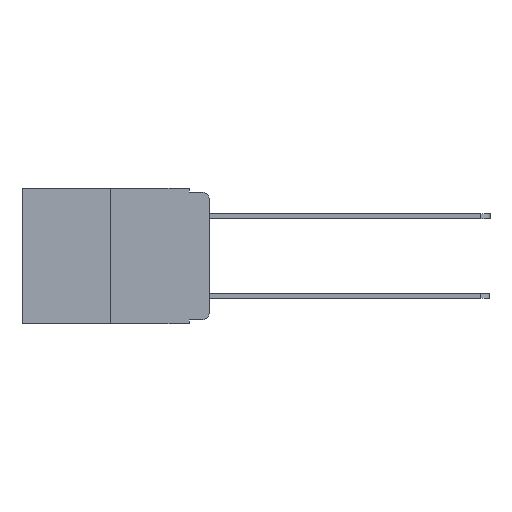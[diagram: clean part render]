
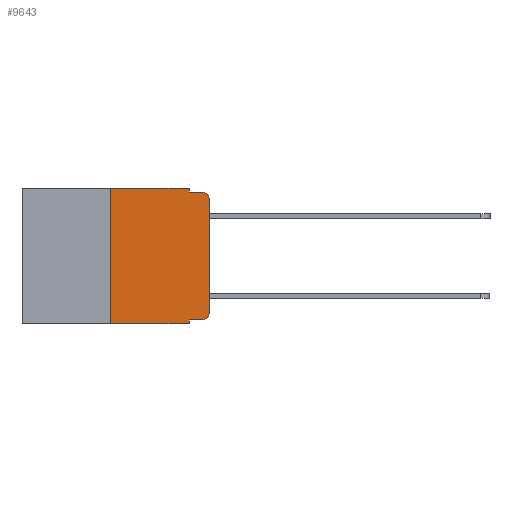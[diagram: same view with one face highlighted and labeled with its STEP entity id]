
A CAD part, left-side view. The second image highlights one B-rep face of the part: STEP entity #9643.
In plain terms, the highlighted planar face has unit normal (-1, 0, 0).
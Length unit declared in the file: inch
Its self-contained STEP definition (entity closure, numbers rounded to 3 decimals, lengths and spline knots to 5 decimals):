
#105 = CARTESIAN_POINT ( 'NONE',  ( 0., 0.051, -0.01 ) ) ;
#121 = CARTESIAN_POINT ( 'NONE',  ( 0., 0., -0.03 ) ) ;
#303 = CARTESIAN_POINT ( 'NONE',  ( 0., 0.02, -0.03 ) ) ;
#440 = CARTESIAN_POINT ( 'NONE',  ( 0., 0., -0.313 ) ) ;
#851 = EDGE_CURVE ( 'NONE', #20736, #8374, #11823, .T. ) ;
#1674 = EDGE_CURVE ( 'NONE', #4114, #20736, #7395, .T. ) ;
#1736 = DIRECTION ( 'NONE',  ( 0., 0., 1. ) ) ;
#1778 = AXIS2_PLACEMENT_3D ( 'NONE', #303, #13627, #2288 ) ;
#2103 = DIRECTION ( 'NONE',  ( 0., -1., 0. ) ) ;
#2275 = CARTESIAN_POINT ( 'NONE',  ( 0., 0.051, -0.01 ) ) ;
#2288 = DIRECTION ( 'NONE',  ( 0., 0., -1. ) ) ;
#2421 = ORIENTED_EDGE ( 'NONE', *, *, #851, .T. ) ;
#2631 = DIRECTION ( 'NONE',  ( 0., 0., -1. ) ) ;
#2921 = EDGE_LOOP ( 'NONE', ( #8877, #15632, #22262, #8631, #10680, #23446, #5410, #3330, #23734, #2421 ) ) ;
#2925 = DIRECTION ( 'NONE',  ( 0., -1., 0. ) ) ;
#3235 = CARTESIAN_POINT ( 'NONE',  ( 0., 0.473, 0. ) ) ;
#3330 = ORIENTED_EDGE ( 'NONE', *, *, #20249, .F. ) ;
#3991 = AXIS2_PLACEMENT_3D ( 'NONE', #8422, #21421, #10295 ) ;
#4114 = VERTEX_POINT ( 'NONE', #14947 ) ;
#4833 = CARTESIAN_POINT ( 'NONE',  ( 0., 0.051, 0. ) ) ;
#5077 = CARTESIAN_POINT ( 'NONE',  ( 0., 0.25, -0.343 ) ) ;
#5410 = ORIENTED_EDGE ( 'NONE', *, *, #15609, .T. ) ;
#5533 = VERTEX_POINT ( 'NONE', #17223 ) ;
#6194 = EDGE_CURVE ( 'NONE', #16056, #20361, #22627, .T. ) ;
#6720 = LINE ( 'NONE', #24196, #20964 ) ;
#7053 = CARTESIAN_POINT ( 'NONE',  ( 0., 0.051, -0.343 ) ) ;
#7395 = LINE ( 'NONE', #8939, #17338 ) ;
#8347 = LINE ( 'NONE', #3235, #18231 ) ;
#8374 = VERTEX_POINT ( 'NONE', #440 ) ;
#8422 = CARTESIAN_POINT ( 'NONE',  ( 0., 0.02, -0.313 ) ) ;
#8479 = CARTESIAN_POINT ( 'NONE',  ( 0., 0.25, 0. ) ) ;
#8631 = ORIENTED_EDGE ( 'NONE', *, *, #10132, .F. ) ;
#8759 = FACE_OUTER_BOUND ( 'NONE', #2921, .T. ) ;
#8877 = ORIENTED_EDGE ( 'NONE', *, *, #9950, .T. ) ;
#8939 = CARTESIAN_POINT ( 'NONE',  ( 0., 0.051, -0.333 ) ) ;
#9478 = EDGE_CURVE ( 'NONE', #22803, #20361, #23287, .T. ) ;
#9643 = ADVANCED_FACE ( 'NONE', ( #8759 ), #10147, .F. ) ;
#9950 = EDGE_CURVE ( 'NONE', #8374, #16056, #6720, .T. ) ;
#10132 = EDGE_CURVE ( 'NONE', #5533, #22803, #17490, .T. ) ;
#10147 = PLANE ( 'NONE',  #22801 ) ;
#10295 = DIRECTION ( 'NONE',  ( 0., 0., -1. ) ) ;
#10396 = CARTESIAN_POINT ( 'NONE',  ( 0., 0.02, -0.333 ) ) ;
#10445 = LINE ( 'NONE', #4833, #11604 ) ;
#10680 = ORIENTED_EDGE ( 'NONE', *, *, #22189, .F. ) ;
#10774 = LINE ( 'NONE', #8479, #20094 ) ;
#10908 = EDGE_CURVE ( 'NONE', #18416, #16336, #10774, .T. ) ;
#11604 = VECTOR ( 'NONE', #17900, 39.37008 ) ;
#11823 = CIRCLE ( 'NONE', #3991, 0.02 ) ;
#12043 = CARTESIAN_POINT ( 'NONE',  ( 0., 0.473, 0. ) ) ;
#13627 = DIRECTION ( 'NONE',  ( -1., 0., 0. ) ) ;
#13941 = DIRECTION ( 'NONE',  ( 1., 0., 0. ) ) ;
#14151 = LINE ( 'NONE', #14222, #23360 ) ;
#14222 = CARTESIAN_POINT ( 'NONE',  ( 0., 0.473, -0.343 ) ) ;
#14449 = VERTEX_POINT ( 'NONE', #7053 ) ;
#14947 = CARTESIAN_POINT ( 'NONE',  ( 0., 0.051, -0.333 ) ) ;
#15609 = EDGE_CURVE ( 'NONE', #18416, #14449, #14151, .T. ) ;
#15632 = ORIENTED_EDGE ( 'NONE', *, *, #6194, .T. ) ;
#16005 = DIRECTION ( 'NONE',  ( 0., 0., 1. ) ) ;
#16056 = VERTEX_POINT ( 'NONE', #121 ) ;
#16336 = VERTEX_POINT ( 'NONE', #19913 ) ;
#16909 = VECTOR ( 'NONE', #19164, 39.37008 ) ;
#17223 = CARTESIAN_POINT ( 'NONE',  ( 0., 0.051, 0. ) ) ;
#17245 = VECTOR ( 'NONE', #2103, 39.37008 ) ;
#17338 = VECTOR ( 'NONE', #21941, 39.37008 ) ;
#17490 = LINE ( 'NONE', #21028, #16909 ) ;
#17900 = DIRECTION ( 'NONE',  ( 0., 0., -1. ) ) ;
#18231 = VECTOR ( 'NONE', #23764, 39.37008 ) ;
#18416 = VERTEX_POINT ( 'NONE', #5077 ) ;
#19164 = DIRECTION ( 'NONE',  ( 0., 0., -1. ) ) ;
#19913 = CARTESIAN_POINT ( 'NONE',  ( 0., 0.25, 0. ) ) ;
#20094 = VECTOR ( 'NONE', #16005, 39.37008 ) ;
#20249 = EDGE_CURVE ( 'NONE', #4114, #14449, #10445, .T. ) ;
#20326 = CARTESIAN_POINT ( 'NONE',  ( 0., 0.02, -0.01 ) ) ;
#20361 = VERTEX_POINT ( 'NONE', #20326 ) ;
#20736 = VERTEX_POINT ( 'NONE', #10396 ) ;
#20964 = VECTOR ( 'NONE', #1736, 39.37008 ) ;
#21028 = CARTESIAN_POINT ( 'NONE',  ( 0., 0.051, 0. ) ) ;
#21421 = DIRECTION ( 'NONE',  ( -1., 0., 0. ) ) ;
#21941 = DIRECTION ( 'NONE',  ( 0., -1., 0. ) ) ;
#22189 = EDGE_CURVE ( 'NONE', #16336, #5533, #8347, .T. ) ;
#22262 = ORIENTED_EDGE ( 'NONE', *, *, #9478, .F. ) ;
#22627 = CIRCLE ( 'NONE', #1778, 0.02 ) ;
#22801 = AXIS2_PLACEMENT_3D ( 'NONE', #12043, #13941, #2631 ) ;
#22803 = VERTEX_POINT ( 'NONE', #2275 ) ;
#23287 = LINE ( 'NONE', #105, #17245 ) ;
#23360 = VECTOR ( 'NONE', #2925, 39.37008 ) ;
#23446 = ORIENTED_EDGE ( 'NONE', *, *, #10908, .F. ) ;
#23734 = ORIENTED_EDGE ( 'NONE', *, *, #1674, .T. ) ;
#23764 = DIRECTION ( 'NONE',  ( 0., -1., 0. ) ) ;
#24196 = CARTESIAN_POINT ( 'NONE',  ( 0., 0., 0. ) ) ;
